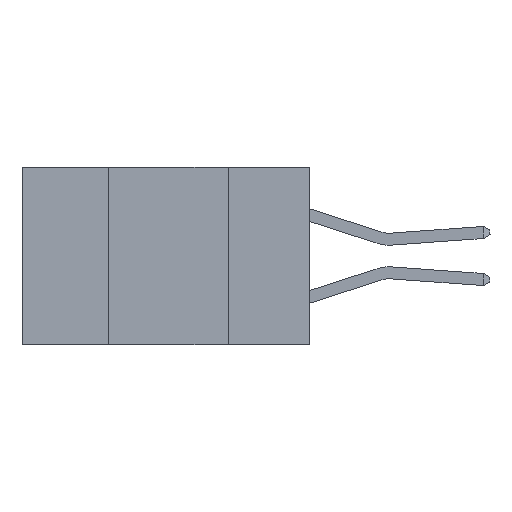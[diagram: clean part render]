
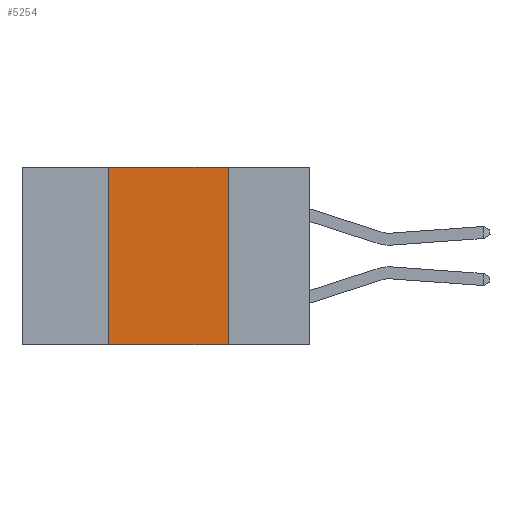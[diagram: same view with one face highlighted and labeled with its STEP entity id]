
A CAD part, left-side view. The second image highlights one B-rep face of the part: STEP entity #5254.
In plain terms, the highlighted planar face has unit normal (-1, 0, 0).
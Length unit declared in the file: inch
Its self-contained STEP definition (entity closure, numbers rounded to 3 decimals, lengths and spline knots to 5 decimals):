
#213 = LINE ( 'NONE', #5722, #9904 ) ;
#362 = PLANE ( 'NONE',  #9239 ) ;
#732 = DIRECTION ( 'NONE',  ( 0., 0., 1. ) ) ;
#815 = VECTOR ( 'NONE', #9132, 39.37008 ) ;
#1112 = FACE_OUTER_BOUND ( 'NONE', #10400, .T. ) ;
#1532 = ORIENTED_EDGE ( 'NONE', *, *, #6160, .T. ) ;
#1617 = CARTESIAN_POINT ( 'NONE',  ( 0., 0.6, 0. ) ) ;
#2566 = ORIENTED_EDGE ( 'NONE', *, *, #11788, .F. ) ;
#3687 = ORIENTED_EDGE ( 'NONE', *, *, #8986, .F. ) ;
#3814 = LINE ( 'NONE', #10085, #6004 ) ;
#3963 = CARTESIAN_POINT ( 'NONE',  ( 0., 0.17, 0. ) ) ;
#5254 = ADVANCED_FACE ( 'NONE', ( #1112 ), #362, .F. ) ;
#5277 = ORIENTED_EDGE ( 'NONE', *, *, #5480, .F. ) ;
#5480 = EDGE_CURVE ( 'NONE', #6397, #8216, #5794, .T. ) ;
#5644 = DIRECTION ( 'NONE',  ( 0., -1., 0. ) ) ;
#5722 = CARTESIAN_POINT ( 'NONE',  ( 0., 0.6, -0.37 ) ) ;
#5794 = LINE ( 'NONE', #1617, #815 ) ;
#5883 = CARTESIAN_POINT ( 'NONE',  ( 0., 0.6, 0. ) ) ;
#5971 = DIRECTION ( 'NONE',  ( 1., 0., 0. ) ) ;
#6004 = VECTOR ( 'NONE', #732, 39.37008 ) ;
#6160 = EDGE_CURVE ( 'NONE', #7860, #7700, #213, .T. ) ;
#6397 = VERTEX_POINT ( 'NONE', #9231 ) ;
#6516 = CARTESIAN_POINT ( 'NONE',  ( 0., 0.17, -0.37 ) ) ;
#7009 = DIRECTION ( 'NONE',  ( 0., 0., -1. ) ) ;
#7276 = VECTOR ( 'NONE', #7009, 39.37008 ) ;
#7700 = VERTEX_POINT ( 'NONE', #6516 ) ;
#7860 = VERTEX_POINT ( 'NONE', #9664 ) ;
#8216 = VERTEX_POINT ( 'NONE', #3963 ) ;
#8986 = EDGE_CURVE ( 'NONE', #7860, #6397, #3814, .T. ) ;
#9132 = DIRECTION ( 'NONE',  ( 0., -1., 0. ) ) ;
#9189 = LINE ( 'NONE', #10759, #7276 ) ;
#9231 = CARTESIAN_POINT ( 'NONE',  ( 0., 0.42, 0. ) ) ;
#9239 = AXIS2_PLACEMENT_3D ( 'NONE', #5883, #5971, #11575 ) ;
#9664 = CARTESIAN_POINT ( 'NONE',  ( 0., 0.42, -0.37 ) ) ;
#9904 = VECTOR ( 'NONE', #5644, 39.37008 ) ;
#10085 = CARTESIAN_POINT ( 'NONE',  ( 0., 0.42, 0. ) ) ;
#10400 = EDGE_LOOP ( 'NONE', ( #2566, #5277, #3687, #1532 ) ) ;
#10759 = CARTESIAN_POINT ( 'NONE',  ( 0., 0.17, 0. ) ) ;
#11575 = DIRECTION ( 'NONE',  ( 0., 0., -1. ) ) ;
#11788 = EDGE_CURVE ( 'NONE', #8216, #7700, #9189, .T. ) ;
